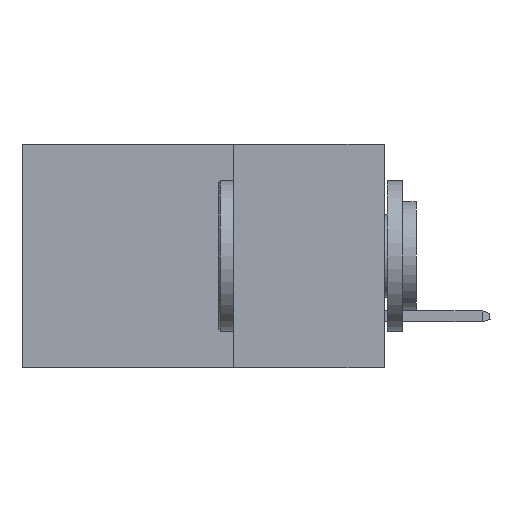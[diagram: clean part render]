
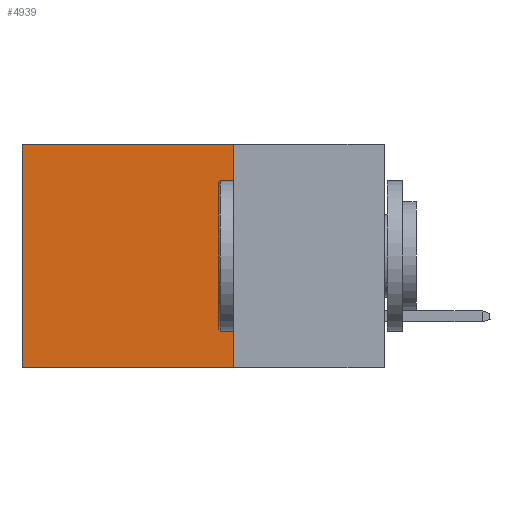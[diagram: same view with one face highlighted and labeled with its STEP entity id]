
A CAD part, left-side view. The second image highlights one B-rep face of the part: STEP entity #4939.
In plain terms, the highlighted planar face has unit normal (-1, 0, 0).
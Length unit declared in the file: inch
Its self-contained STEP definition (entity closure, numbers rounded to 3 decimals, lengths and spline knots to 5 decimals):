
#138 = EDGE_CURVE ( 'NONE', #11454, #2222, #2046, .T. ) ;
#386 = ORIENTED_EDGE ( 'NONE', *, *, #14220, .F. ) ;
#736 = FACE_OUTER_BOUND ( 'NONE', #7308, .T. ) ;
#1371 = VECTOR ( 'NONE', #10474, 39.37008 ) ;
#2046 = LINE ( 'NONE', #15226, #8916 ) ;
#2222 = VERTEX_POINT ( 'NONE', #11432 ) ;
#3440 = CARTESIAN_POINT ( 'NONE',  ( 0.298, 0.6, 0. ) ) ;
#3516 = DIRECTION ( 'NONE',  ( 1., 0., 0. ) ) ;
#3718 = ORIENTED_EDGE ( 'NONE', *, *, #10660, .T. ) ;
#3738 = CARTESIAN_POINT ( 'NONE',  ( 0.298, 0.25, 0. ) ) ;
#3884 = LINE ( 'NONE', #14840, #8327 ) ;
#4939 = ADVANCED_FACE ( 'NONE', ( #736 ), #9178, .F. ) ;
#6368 = CARTESIAN_POINT ( 'NONE',  ( 0.298, 0.6, -0.37 ) ) ;
#7155 = LINE ( 'NONE', #3440, #1371 ) ;
#7308 = EDGE_LOOP ( 'NONE', ( #3718, #386, #15022, #13305 ) ) ;
#7886 = VECTOR ( 'NONE', #14382, 39.37008 ) ;
#8327 = VECTOR ( 'NONE', #14993, 39.37008 ) ;
#8807 = LINE ( 'NONE', #3738, #7886 ) ;
#8916 = VECTOR ( 'NONE', #11718, 39.37008 ) ;
#9178 = PLANE ( 'NONE',  #11795 ) ;
#9368 = VERTEX_POINT ( 'NONE', #6368 ) ;
#9532 = VERTEX_POINT ( 'NONE', #10544 ) ;
#10474 = DIRECTION ( 'NONE',  ( 0., 0., -1. ) ) ;
#10488 = EDGE_CURVE ( 'NONE', #11454, #9532, #8807, .T. ) ;
#10544 = CARTESIAN_POINT ( 'NONE',  ( 0.298, 0.25, -0.37 ) ) ;
#10660 = EDGE_CURVE ( 'NONE', #2222, #9368, #7155, .T. ) ;
#11432 = CARTESIAN_POINT ( 'NONE',  ( 0.298, 0.6, 0. ) ) ;
#11454 = VERTEX_POINT ( 'NONE', #14126 ) ;
#11718 = DIRECTION ( 'NONE',  ( 0., 1., 0. ) ) ;
#11795 = AXIS2_PLACEMENT_3D ( 'NONE', #13926, #3516, #13025 ) ;
#13025 = DIRECTION ( 'NONE',  ( 0., 0., -1. ) ) ;
#13305 = ORIENTED_EDGE ( 'NONE', *, *, #138, .T. ) ;
#13926 = CARTESIAN_POINT ( 'NONE',  ( 0.298, 0.25, 0. ) ) ;
#14126 = CARTESIAN_POINT ( 'NONE',  ( 0.298, 0.25, 0. ) ) ;
#14220 = EDGE_CURVE ( 'NONE', #9532, #9368, #3884, .T. ) ;
#14382 = DIRECTION ( 'NONE',  ( 0., 0., -1. ) ) ;
#14840 = CARTESIAN_POINT ( 'NONE',  ( 0.298, 0.25, -0.37 ) ) ;
#14993 = DIRECTION ( 'NONE',  ( 0., 1., 0. ) ) ;
#15022 = ORIENTED_EDGE ( 'NONE', *, *, #10488, .F. ) ;
#15226 = CARTESIAN_POINT ( 'NONE',  ( 0.298, 0.25, 0. ) ) ;
